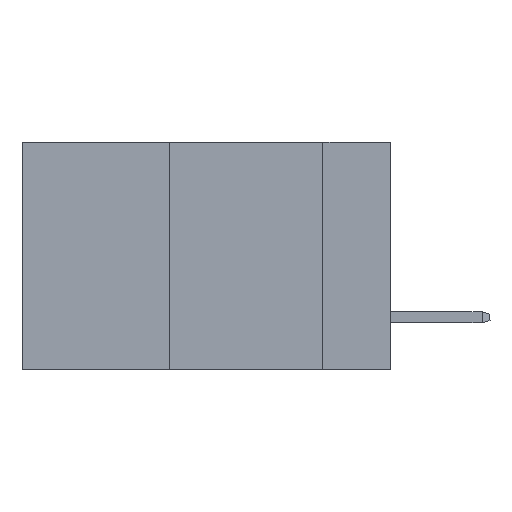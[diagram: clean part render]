
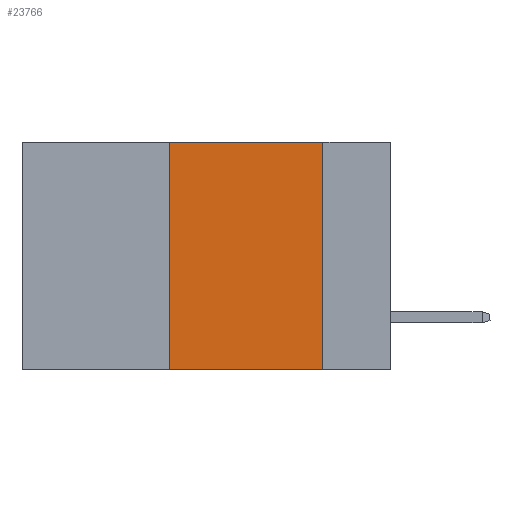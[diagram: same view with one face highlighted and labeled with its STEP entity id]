
A CAD part, left-side view. The second image highlights one B-rep face of the part: STEP entity #23766.
In plain terms, the highlighted planar face has unit normal (-1, 0, 0).
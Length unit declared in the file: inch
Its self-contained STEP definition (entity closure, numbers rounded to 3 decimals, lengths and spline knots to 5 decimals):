
#216 = VERTEX_POINT ( 'NONE', #18945 ) ;
#476 = DIRECTION ( 'NONE',  ( 1., 0., 0. ) ) ;
#638 = DIRECTION ( 'NONE',  ( 0., -1., 0. ) ) ;
#1219 = ORIENTED_EDGE ( 'NONE', *, *, #17038, .F. ) ;
#1379 = FACE_OUTER_BOUND ( 'NONE', #8255, .T. ) ;
#3503 = VECTOR ( 'NONE', #30760, 39.37008 ) ;
#6810 = VERTEX_POINT ( 'NONE', #34089 ) ;
#6818 = LINE ( 'NONE', #12246, #35070 ) ;
#8255 = EDGE_LOOP ( 'NONE', ( #1219, #22656, #10600, #28637 ) ) ;
#8446 = CARTESIAN_POINT ( 'NONE',  ( 0., 0.11, 0. ) ) ;
#8921 = CARTESIAN_POINT ( 'NONE',  ( 0., 0.6, 0. ) ) ;
#10600 = ORIENTED_EDGE ( 'NONE', *, *, #25044, .F. ) ;
#11716 = CARTESIAN_POINT ( 'NONE',  ( 0., 0.36, 0. ) ) ;
#12246 = CARTESIAN_POINT ( 'NONE',  ( 0., 0.6, -0.37 ) ) ;
#12674 = CARTESIAN_POINT ( 'NONE',  ( 0., 0.11, -0.37 ) ) ;
#15879 = EDGE_CURVE ( 'NONE', #6810, #31185, #6818, .T. ) ;
#17038 = EDGE_CURVE ( 'NONE', #21900, #31185, #24781, .T. ) ;
#17050 = CARTESIAN_POINT ( 'NONE',  ( 0., 0.6, 0. ) ) ;
#17973 = LINE ( 'NONE', #8921, #24388 ) ;
#18945 = CARTESIAN_POINT ( 'NONE',  ( 0., 0.36, 0. ) ) ;
#19794 = DIRECTION ( 'NONE',  ( 0., 0., -1. ) ) ;
#21900 = VERTEX_POINT ( 'NONE', #8446 ) ;
#22004 = EDGE_CURVE ( 'NONE', #216, #21900, #17973, .T. ) ;
#22656 = ORIENTED_EDGE ( 'NONE', *, *, #22004, .F. ) ;
#23024 = DIRECTION ( 'NONE',  ( 0., 0., -1. ) ) ;
#23766 = ADVANCED_FACE ( 'NONE', ( #1379 ), #27936, .F. ) ;
#24388 = VECTOR ( 'NONE', #638, 39.37008 ) ;
#24639 = LINE ( 'NONE', #11716, #3503 ) ;
#24781 = LINE ( 'NONE', #31103, #31128 ) ;
#25044 = EDGE_CURVE ( 'NONE', #6810, #216, #24639, .T. ) ;
#25981 = DIRECTION ( 'NONE',  ( 0., -1., 0. ) ) ;
#27936 = PLANE ( 'NONE',  #33037 ) ;
#28637 = ORIENTED_EDGE ( 'NONE', *, *, #15879, .T. ) ;
#30760 = DIRECTION ( 'NONE',  ( 0., 0., 1. ) ) ;
#31103 = CARTESIAN_POINT ( 'NONE',  ( 0., 0.11, 0. ) ) ;
#31128 = VECTOR ( 'NONE', #23024, 39.37008 ) ;
#31185 = VERTEX_POINT ( 'NONE', #12674 ) ;
#33037 = AXIS2_PLACEMENT_3D ( 'NONE', #17050, #476, #19794 ) ;
#34089 = CARTESIAN_POINT ( 'NONE',  ( 0., 0.36, -0.37 ) ) ;
#35070 = VECTOR ( 'NONE', #25981, 39.37008 ) ;
